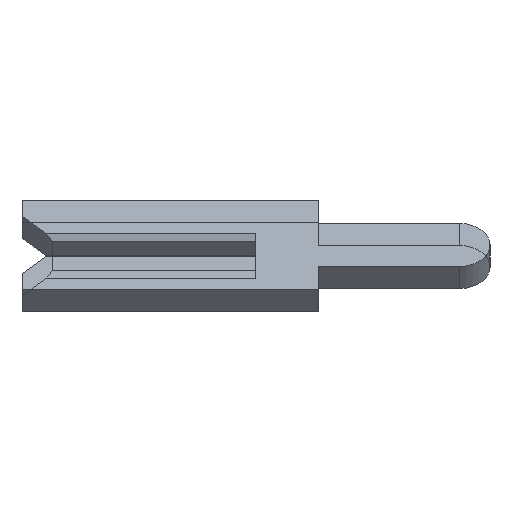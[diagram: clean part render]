
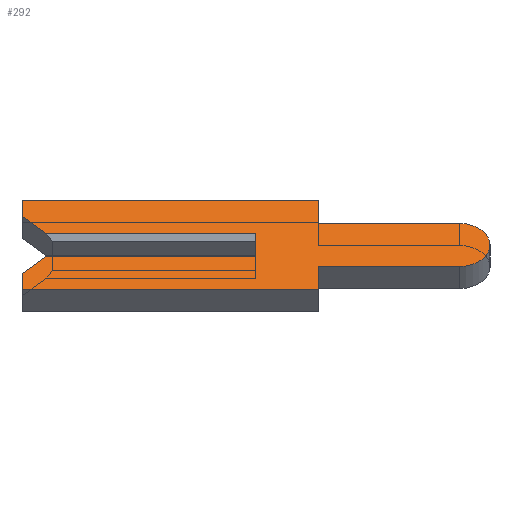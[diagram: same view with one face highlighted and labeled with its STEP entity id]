
A CAD part, left-side view. The second image highlights one B-rep face of the part: STEP entity #292.
In plain terms, the highlighted face is planar.
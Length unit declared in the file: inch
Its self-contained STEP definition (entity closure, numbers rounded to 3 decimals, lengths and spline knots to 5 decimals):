
#51 = VERTEX_POINT ( 'NONE', #3186 ) ;
#53 = DIRECTION ( 'NONE',  ( 0., 1., 0. ) ) ;
#72 = DIRECTION ( 'NONE',  ( 0., 0., -1. ) ) ;
#80 = CARTESIAN_POINT ( 'NONE',  ( -0.01, 0.15, -0.026 ) ) ;
#109 = CARTESIAN_POINT ( 'NONE',  ( -0.01, -0.1305, 0. ) ) ;
#132 = VECTOR ( 'NONE', #1236, 39.37008 ) ;
#185 = EDGE_CURVE ( 'NONE', #1130, #2758, #2138, .T. ) ;
#189 = VECTOR ( 'NONE', #53, 39.37008 ) ;
#198 = CARTESIAN_POINT ( 'NONE',  ( -0.01, -0.1305, -0.0195 ) ) ;
#231 = DIRECTION ( 'NONE',  ( 0., 0., -1. ) ) ;
#232 = ORIENTED_EDGE ( 'NONE', *, *, #3674, .F. ) ;
#292 = ADVANCED_FACE ( 'NONE', ( #1322 ), #1830, .F. ) ;
#341 = LINE ( 'NONE', #797, #3524 ) ;
#396 = DIRECTION ( 'NONE',  ( 0., -1., 0. ) ) ;
#442 = DIRECTION ( 'NONE',  ( 1., 0., 0. ) ) ;
#447 = VECTOR ( 'NONE', #745, 39.37008 ) ;
#456 = CARTESIAN_POINT ( 'NONE',  ( -0.01, 0.15, 0.04 ) ) ;
#482 = ORIENTED_EDGE ( 'NONE', *, *, #1607, .F. ) ;
#484 = CARTESIAN_POINT ( 'NONE',  ( -0.01, 0.1305, -0.0065 ) ) ;
#510 = DIRECTION ( 'NONE',  ( 0., -0.707, 0.707 ) ) ;
#532 = DIRECTION ( 'NONE',  ( 1., 0., 0. ) ) ;
#560 = CARTESIAN_POINT ( 'NONE',  ( -0.01, 0.1305, 0.0065 ) ) ;
#583 = CARTESIAN_POINT ( 'NONE',  ( -0.01, -0.04, -0.0195 ) ) ;
#587 = VERTEX_POINT ( 'NONE', #2401 ) ;
#606 = ORIENTED_EDGE ( 'NONE', *, *, #708, .F. ) ;
#708 = EDGE_CURVE ( 'NONE', #3353, #827, #1654, .T. ) ;
#745 = DIRECTION ( 'NONE',  ( 0., -1., 0. ) ) ;
#761 = LINE ( 'NONE', #3440, #4223 ) ;
#797 = CARTESIAN_POINT ( 'NONE',  ( -0.01, -0.04, 0.0195 ) ) ;
#801 = ORIENTED_EDGE ( 'NONE', *, *, #1121, .T. ) ;
#827 = VERTEX_POINT ( 'NONE', #3414 ) ;
#937 = LINE ( 'NONE', #2339, #3460 ) ;
#952 = EDGE_CURVE ( 'NONE', #2648, #587, #761, .T. ) ;
#965 = ORIENTED_EDGE ( 'NONE', *, *, #2893, .F. ) ;
#1075 = LINE ( 'NONE', #560, #4069 ) ;
#1108 = VERTEX_POINT ( 'NONE', #2832 ) ;
#1117 = CARTESIAN_POINT ( 'NONE',  ( -0.01, 0.15, 0.026 ) ) ;
#1121 = EDGE_CURVE ( 'NONE', #51, #587, #2402, .T. ) ;
#1130 = VERTEX_POINT ( 'NONE', #3176 ) ;
#1192 = EDGE_LOOP ( 'NONE', ( #801, #3235, #2227, #3722, #3415, #1299, #232, #2254, #1955, #3994, #606, #482, #2750, #965 ) ) ;
#1236 = DIRECTION ( 'NONE',  ( 0., 0., 1. ) ) ;
#1253 = VERTEX_POINT ( 'NONE', #3556 ) ;
#1276 = EDGE_CURVE ( 'NONE', #2950, #2632, #2884, .T. ) ;
#1299 = ORIENTED_EDGE ( 'NONE', *, *, #1501, .F. ) ;
#1322 = FACE_OUTER_BOUND ( 'NONE', #1192, .T. ) ;
#1323 = CARTESIAN_POINT ( 'NONE',  ( -0.01, -0.04, -0.0195 ) ) ;
#1386 = CARTESIAN_POINT ( 'NONE',  ( -0.01, -0.04, 0.04 ) ) ;
#1400 = VERTEX_POINT ( 'NONE', #1117 ) ;
#1426 = VECTOR ( 'NONE', #510, 39.37008 ) ;
#1486 = DIRECTION ( 'NONE',  ( 0., 0., 1. ) ) ;
#1494 = CARTESIAN_POINT ( 'NONE',  ( -0.01, -0.1305, 0. ) ) ;
#1501 = EDGE_CURVE ( 'NONE', #3775, #1130, #1802, .T. ) ;
#1543 = LINE ( 'NONE', #456, #3265 ) ;
#1562 = CARTESIAN_POINT ( 'NONE',  ( -0.01, 0., -0.01 ) ) ;
#1607 = EDGE_CURVE ( 'NONE', #1108, #3353, #1543, .T. ) ;
#1654 = LINE ( 'NONE', #1386, #2620 ) ;
#1660 = CARTESIAN_POINT ( 'NONE',  ( -0.01, -0.04, -0.04 ) ) ;
#1767 = AXIS2_PLACEMENT_3D ( 'NONE', #1494, #442, #72 ) ;
#1802 = LINE ( 'NONE', #3833, #189 ) ;
#1830 = PLANE ( 'NONE',  #4185 ) ;
#1917 = LINE ( 'NONE', #484, #1426 ) ;
#1921 = VECTOR ( 'NONE', #1486, 39.37008 ) ;
#1955 = ORIENTED_EDGE ( 'NONE', *, *, #1276, .F. ) ;
#1981 = EDGE_CURVE ( 'NONE', #827, #2950, #341, .T. ) ;
#2036 = CARTESIAN_POINT ( 'NONE',  ( -0.01, -0.1305, -0.01 ) ) ;
#2138 = LINE ( 'NONE', #80, #1921 ) ;
#2192 = LINE ( 'NONE', #2613, #132 ) ;
#2227 = ORIENTED_EDGE ( 'NONE', *, *, #4070, .F. ) ;
#2254 = ORIENTED_EDGE ( 'NONE', *, *, #3954, .F. ) ;
#2307 = EDGE_CURVE ( 'NONE', #2758, #1253, #1917, .T. ) ;
#2339 = CARTESIAN_POINT ( 'NONE',  ( -0.01, -0.04, -0.04 ) ) ;
#2401 = CARTESIAN_POINT ( 'NONE',  ( -0.01, 0., 0.01 ) ) ;
#2402 = LINE ( 'NONE', #3523, #447 ) ;
#2613 = CARTESIAN_POINT ( 'NONE',  ( -0.01, 0.15, 0.026 ) ) ;
#2620 = VECTOR ( 'NONE', #231, 39.37008 ) ;
#2632 = VERTEX_POINT ( 'NONE', #198 ) ;
#2648 = VERTEX_POINT ( 'NONE', #1562 ) ;
#2750 = ORIENTED_EDGE ( 'NONE', *, *, #2913, .F. ) ;
#2758 = VERTEX_POINT ( 'NONE', #2978 ) ;
#2832 = CARTESIAN_POINT ( 'NONE',  ( -0.01, 0.15, 0.04 ) ) ;
#2884 = CIRCLE ( 'NONE', #1767, 0.0195 ) ;
#2893 = EDGE_CURVE ( 'NONE', #51, #1400, #1075, .T. ) ;
#2913 = EDGE_CURVE ( 'NONE', #1400, #1108, #2192, .T. ) ;
#2935 = VERTEX_POINT ( 'NONE', #583 ) ;
#2950 = VERTEX_POINT ( 'NONE', #3347 ) ;
#2978 = CARTESIAN_POINT ( 'NONE',  ( -0.01, 0.15, -0.026 ) ) ;
#2992 = DIRECTION ( 'NONE',  ( 0., 0.707, 0.707 ) ) ;
#3018 = CARTESIAN_POINT ( 'NONE',  ( -0.01, -0.04, 0.04 ) ) ;
#3047 = DIRECTION ( 'NONE',  ( 0., -1., 0. ) ) ;
#3054 = DIRECTION ( 'NONE',  ( 0., 0., -1. ) ) ;
#3088 = LINE ( 'NONE', #2036, #3693 ) ;
#3127 = DIRECTION ( 'NONE',  ( 0., 0., 1. ) ) ;
#3176 = CARTESIAN_POINT ( 'NONE',  ( -0.01, 0.15, -0.04 ) ) ;
#3186 = CARTESIAN_POINT ( 'NONE',  ( -0.01, 0.134, 0.01 ) ) ;
#3204 = LINE ( 'NONE', #1323, #3354 ) ;
#3235 = ORIENTED_EDGE ( 'NONE', *, *, #952, .F. ) ;
#3265 = VECTOR ( 'NONE', #396, 39.37008 ) ;
#3285 = DIRECTION ( 'NONE',  ( 0., -1., 0. ) ) ;
#3347 = CARTESIAN_POINT ( 'NONE',  ( -0.01, -0.1305, 0.0195 ) ) ;
#3353 = VERTEX_POINT ( 'NONE', #3018 ) ;
#3354 = VECTOR ( 'NONE', #3394, 39.37008 ) ;
#3394 = DIRECTION ( 'NONE',  ( 0., 1., 0. ) ) ;
#3414 = CARTESIAN_POINT ( 'NONE',  ( -0.01, -0.04, 0.0195 ) ) ;
#3415 = ORIENTED_EDGE ( 'NONE', *, *, #185, .F. ) ;
#3440 = CARTESIAN_POINT ( 'NONE',  ( -0.01, 0., 0.0065 ) ) ;
#3460 = VECTOR ( 'NONE', #3054, 39.37008 ) ;
#3523 = CARTESIAN_POINT ( 'NONE',  ( -0.01, 0.15, 0.01 ) ) ;
#3524 = VECTOR ( 'NONE', #3285, 39.37008 ) ;
#3556 = CARTESIAN_POINT ( 'NONE',  ( -0.01, 0.134, -0.01 ) ) ;
#3674 = EDGE_CURVE ( 'NONE', #2935, #3775, #937, .T. ) ;
#3693 = VECTOR ( 'NONE', #3047, 39.37008 ) ;
#3722 = ORIENTED_EDGE ( 'NONE', *, *, #2307, .F. ) ;
#3764 = DIRECTION ( 'NONE',  ( 0., 0., -1. ) ) ;
#3775 = VERTEX_POINT ( 'NONE', #1660 ) ;
#3833 = CARTESIAN_POINT ( 'NONE',  ( -0.01, 0.15, -0.04 ) ) ;
#3954 = EDGE_CURVE ( 'NONE', #2632, #2935, #3204, .T. ) ;
#3994 = ORIENTED_EDGE ( 'NONE', *, *, #1981, .F. ) ;
#4069 = VECTOR ( 'NONE', #2992, 39.37008 ) ;
#4070 = EDGE_CURVE ( 'NONE', #1253, #2648, #3088, .T. ) ;
#4185 = AXIS2_PLACEMENT_3D ( 'NONE', #109, #532, #3764 ) ;
#4223 = VECTOR ( 'NONE', #3127, 39.37008 ) ;
